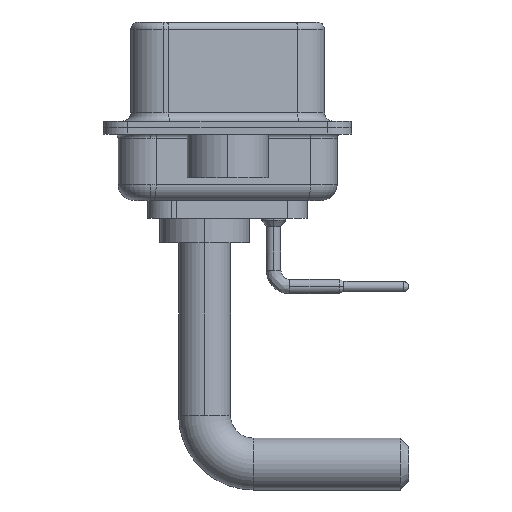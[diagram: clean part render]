
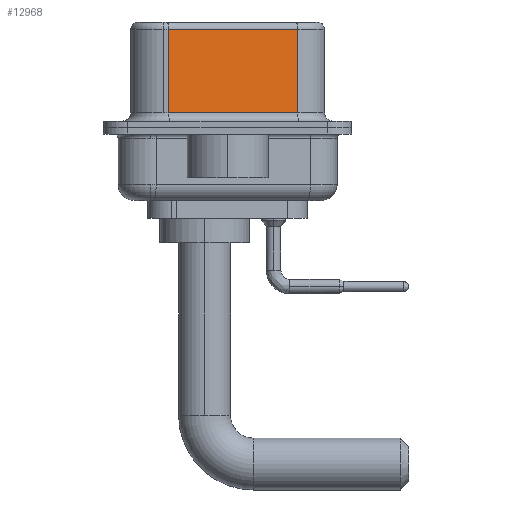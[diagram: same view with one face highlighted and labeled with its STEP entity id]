
A CAD part, left-side view. The second image highlights one B-rep face of the part: STEP entity #12968.
In plain terms, the highlighted planar face has unit normal (-0.985, -0.174, 0).
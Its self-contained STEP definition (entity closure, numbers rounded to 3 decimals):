
#494 = EDGE_CURVE ( 'NONE', #17508, #527, #19799, .T. ) ;
#527 = VERTEX_POINT ( 'NONE', #20039 ) ;
#574 = ORIENTED_EDGE ( 'NONE', *, *, #19340, .F. ) ;
#890 = EDGE_CURVE ( 'NONE', #10247, #17508, #12394, .T. ) ;
#2589 = DIRECTION ( 'NONE',  ( 0.985, 0.174, 0. ) ) ;
#4243 = ORIENTED_EDGE ( 'NONE', *, *, #890, .T. ) ;
#4690 = DIRECTION ( 'NONE',  ( 0., 0., -1. ) ) ;
#5565 = LINE ( 'NONE', #7252, #19537 ) ;
#6113 = DIRECTION ( 'NONE',  ( 0.174, -0.985, 0. ) ) ;
#6226 = CARTESIAN_POINT ( 'NONE',  ( 5.132, -4.322, 0.9 ) ) ;
#7252 = CARTESIAN_POINT ( 'NONE',  ( 5.132, -4.322, 6.52 ) ) ;
#8137 = DIRECTION ( 'NONE',  ( -0.174, 0.985, 0. ) ) ;
#8619 = FACE_OUTER_BOUND ( 'NONE', #10341, .T. ) ;
#10247 = VERTEX_POINT ( 'NONE', #18050 ) ;
#10341 = EDGE_LOOP ( 'NONE', ( #574, #4243, #11375, #13993 ) ) ;
#10464 = CARTESIAN_POINT ( 'NONE',  ( 5.132, -4.322, 6.02 ) ) ;
#10750 = EDGE_CURVE ( 'NONE', #527, #23246, #15186, .T. ) ;
#11375 = ORIENTED_EDGE ( 'NONE', *, *, #494, .T. ) ;
#11764 = CARTESIAN_POINT ( 'NONE',  ( 5.132, -4.322, 6.52 ) ) ;
#12394 = LINE ( 'NONE', #10464, #13567 ) ;
#12968 = ADVANCED_FACE ( 'NONE', ( #8619 ), #21561, .F. ) ;
#13567 = VECTOR ( 'NONE', #13717, 1000. ) ;
#13717 = DIRECTION ( 'NONE',  ( -0.174, 0.985, 0. ) ) ;
#13993 = ORIENTED_EDGE ( 'NONE', *, *, #10750, .T. ) ;
#14794 = VECTOR ( 'NONE', #4690, 1000. ) ;
#15186 = LINE ( 'NONE', #6226, #16328 ) ;
#15935 = CARTESIAN_POINT ( 'NONE',  ( 3.73, 3.628, 6.52 ) ) ;
#16328 = VECTOR ( 'NONE', #6113, 1000. ) ;
#17508 = VERTEX_POINT ( 'NONE', #18641 ) ;
#17999 = CARTESIAN_POINT ( 'NONE',  ( 5.132, -4.322, 0.9 ) ) ;
#18050 = CARTESIAN_POINT ( 'NONE',  ( 5.132, -4.322, 6.02 ) ) ;
#18641 = CARTESIAN_POINT ( 'NONE',  ( 3.73, 3.628, 6.02 ) ) ;
#19340 = EDGE_CURVE ( 'NONE', #10247, #23246, #5565, .T. ) ;
#19537 = VECTOR ( 'NONE', #20302, 1000. ) ;
#19799 = LINE ( 'NONE', #15935, #14794 ) ;
#20039 = CARTESIAN_POINT ( 'NONE',  ( 3.73, 3.628, 0.9 ) ) ;
#20302 = DIRECTION ( 'NONE',  ( 0., 0., -1. ) ) ;
#20624 = AXIS2_PLACEMENT_3D ( 'NONE', #11764, #2589, #8137 ) ;
#21561 = PLANE ( 'NONE',  #20624 ) ;
#23246 = VERTEX_POINT ( 'NONE', #17999 ) ;
